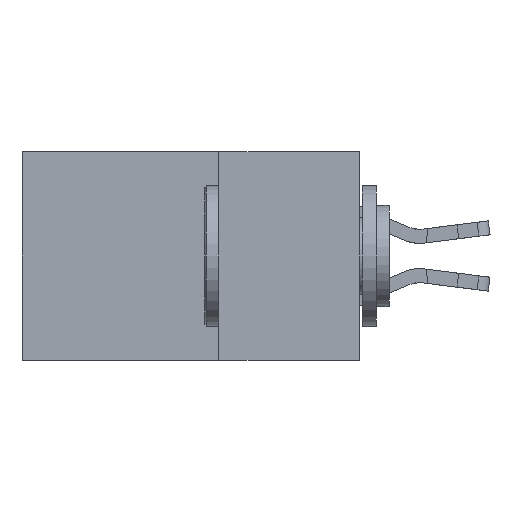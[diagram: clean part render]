
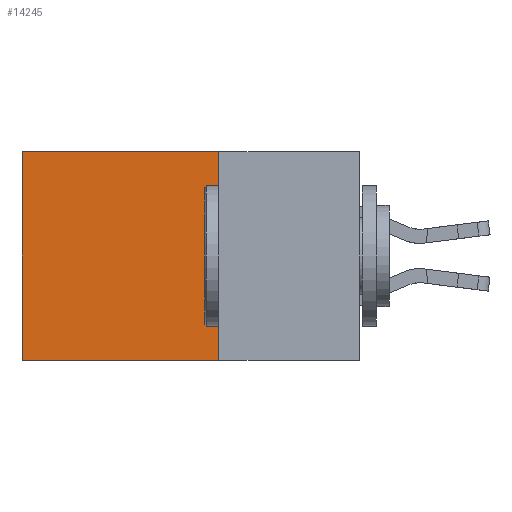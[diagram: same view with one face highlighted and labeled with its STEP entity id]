
A CAD part, left-side view. The second image highlights one B-rep face of the part: STEP entity #14245.
In plain terms, the highlighted planar face has unit normal (-1, 0, 0).
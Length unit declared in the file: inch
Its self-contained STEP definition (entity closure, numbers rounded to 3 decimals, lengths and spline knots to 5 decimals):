
#2141 = FACE_OUTER_BOUND ( 'NONE', #14975, .T. ) ;
#4594 = LINE ( 'NONE', #21012, #12316 ) ;
#5195 = VERTEX_POINT ( 'NONE', #22323 ) ;
#5382 = LINE ( 'NONE', #18387, #23155 ) ;
#5628 = ORIENTED_EDGE ( 'NONE', *, *, #19446, .T. ) ;
#5945 = CARTESIAN_POINT ( 'NONE',  ( 0.2875, 0.25, 0. ) ) ;
#6476 = DIRECTION ( 'NONE',  ( 0., 1., 0. ) ) ;
#7140 = DIRECTION ( 'NONE',  ( 0., 0., -1. ) ) ;
#7225 = DIRECTION ( 'NONE',  ( 0., 0., -1. ) ) ;
#8925 = VERTEX_POINT ( 'NONE', #22462 ) ;
#10330 = EDGE_CURVE ( 'NONE', #5195, #25652, #5382, .T. ) ;
#11442 = LINE ( 'NONE', #20391, #29724 ) ;
#12316 = VECTOR ( 'NONE', #7140, 39.37008 ) ;
#14245 = ADVANCED_FACE ( 'NONE', ( #2141 ), #16472, .F. ) ;
#14975 = EDGE_LOOP ( 'NONE', ( #17114, #19944, #25830, #5628 ) ) ;
#15500 = AXIS2_PLACEMENT_3D ( 'NONE', #18788, #21096, #7225 ) ;
#16164 = CARTESIAN_POINT ( 'NONE',  ( 0.2875, 0.25, 0. ) ) ;
#16472 = PLANE ( 'NONE',  #15500 ) ;
#16477 = EDGE_CURVE ( 'NONE', #16956, #8925, #4594, .T. ) ;
#16818 = VECTOR ( 'NONE', #22163, 39.37008 ) ;
#16956 = VERTEX_POINT ( 'NONE', #16164 ) ;
#17114 = ORIENTED_EDGE ( 'NONE', *, *, #10330, .T. ) ;
#18387 = CARTESIAN_POINT ( 'NONE',  ( 0.2875, 0.6, 0. ) ) ;
#18788 = CARTESIAN_POINT ( 'NONE',  ( 0.2875, 0.25, 0. ) ) ;
#18966 = EDGE_CURVE ( 'NONE', #8925, #25652, #11442, .T. ) ;
#19446 = EDGE_CURVE ( 'NONE', #16956, #5195, #22210, .T. ) ;
#19944 = ORIENTED_EDGE ( 'NONE', *, *, #18966, .F. ) ;
#20391 = CARTESIAN_POINT ( 'NONE',  ( 0.2875, 0.25, -0.37 ) ) ;
#20700 = DIRECTION ( 'NONE',  ( 0., 0., -1. ) ) ;
#21012 = CARTESIAN_POINT ( 'NONE',  ( 0.2875, 0.25, 0. ) ) ;
#21096 = DIRECTION ( 'NONE',  ( 1., 0., 0. ) ) ;
#22163 = DIRECTION ( 'NONE',  ( 0., 1., 0. ) ) ;
#22210 = LINE ( 'NONE', #5945, #16818 ) ;
#22323 = CARTESIAN_POINT ( 'NONE',  ( 0.2875, 0.6, 0. ) ) ;
#22462 = CARTESIAN_POINT ( 'NONE',  ( 0.2875, 0.25, -0.37 ) ) ;
#22503 = CARTESIAN_POINT ( 'NONE',  ( 0.2875, 0.6, -0.37 ) ) ;
#23155 = VECTOR ( 'NONE', #20700, 39.37008 ) ;
#25652 = VERTEX_POINT ( 'NONE', #22503 ) ;
#25830 = ORIENTED_EDGE ( 'NONE', *, *, #16477, .F. ) ;
#29724 = VECTOR ( 'NONE', #6476, 39.37008 ) ;
